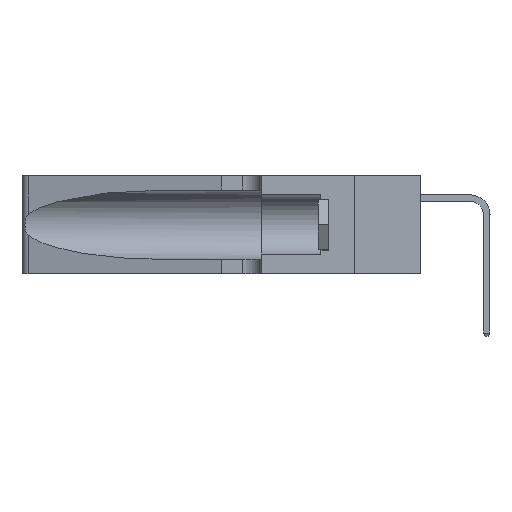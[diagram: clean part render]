
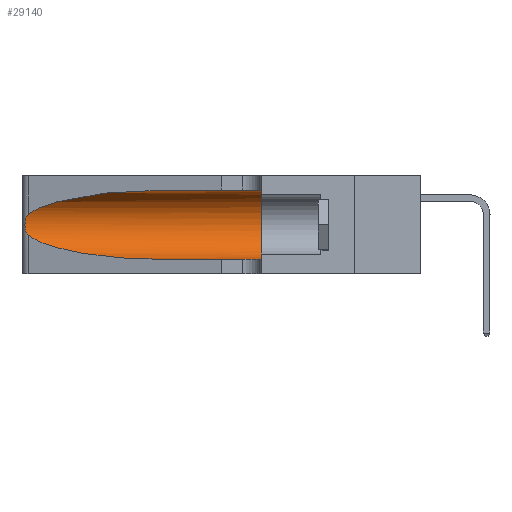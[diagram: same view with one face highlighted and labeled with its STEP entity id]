
A CAD part, left-side view. The second image highlights one B-rep face of the part: STEP entity #29140.
In plain terms, the highlighted cylindrical face has radius 3.308 mm (diameter 6.617 mm), a partial arc.
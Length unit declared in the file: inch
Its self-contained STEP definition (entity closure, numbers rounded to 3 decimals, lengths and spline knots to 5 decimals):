
#673 = CARTESIAN_POINT ( 'NONE',  ( 0.25487, 1.22718, 0.14631 ) ) ;
#947 = ORIENTED_EDGE ( 'NONE', *, *, #42946, .T. ) ;
#1863 = CARTESIAN_POINT ( 'NONE',  ( 0.1305, 0.35, 0.185 ) ) ;
#2248 = CARTESIAN_POINT ( 'NONE',  ( 0.25487, 1.22718, 0.22369 ) ) ;
#2252 = ORIENTED_EDGE ( 'NONE', *, *, #33688, .F. ) ;
#2518 = CARTESIAN_POINT ( 'NONE',  ( 0.1305, 1.61858, 0.05475 ) ) ;
#2894 = CARTESIAN_POINT ( 'NONE',  ( 0.18966, 0.96281, 0.31525 ) ) ;
#3070 = AXIS2_PLACEMENT_3D ( 'NONE', #3929, #15166, #40957 ) ;
#3604 = CARTESIAN_POINT ( 'NONE',  ( 0.26017, 1.23833, 0.17102 ) ) ;
#3897 = ORIENTED_EDGE ( 'NONE', *, *, #32656, .T. ) ;
#3929 = CARTESIAN_POINT ( 'NONE',  ( 0.1305, 1.61858, 0.185 ) ) ;
#5640 = DIRECTION ( 'NONE',  ( 0., 0., 1. ) ) ;
#5863 =( BOUNDED_CURVE ( )  B_SPLINE_CURVE ( 3, ( #28818, #2894, #32540, #10433 ),
 .UNSPECIFIED., .F., .T. ) 
 B_SPLINE_CURVE_WITH_KNOTS ( ( 4, 4 ),
 ( 1.5708, 2.84003 ),
 .UNSPECIFIED. ) 
 CURVE ( )  GEOMETRIC_REPRESENTATION_ITEM ( )  RATIONAL_B_SPLINE_CURVE ( ( 1., 0.87, 0.87, 1. ) ) 
 REPRESENTATION_ITEM ( '' )  );
#6295 = DIRECTION ( 'NONE',  ( 0., -1., 0. ) ) ;
#6692 = ORIENTED_EDGE ( 'NONE', *, *, #34399, .F. ) ;
#6877 = EDGE_CURVE ( 'NONE', #47892, #19113, #18857, .T. ) ;
#7237 = CARTESIAN_POINT ( 'NONE',  ( 0.25555, 1.22994, 0.2215 ) ) ;
#7405 = CARTESIAN_POINT ( 'NONE',  ( 0.25789, 1.23486, 0.15765 ) ) ;
#8239 = CARTESIAN_POINT ( 'NONE',  ( 0.1305, 0.72297, 0.05475 ) ) ;
#9835 = CARTESIAN_POINT ( 'NONE',  ( 0.1305, 1.61858, 0.31525 ) ) ;
#9887 = VECTOR ( 'NONE', #13546, 39.37008 ) ;
#10189 = EDGE_CURVE ( 'NONE', #40850, #20767, #39836, .T. ) ;
#10433 = CARTESIAN_POINT ( 'NONE',  ( 0.25487, 1.22718, 0.22369 ) ) ;
#11052 = LINE ( 'NONE', #9835, #9887 ) ;
#11140 = CARTESIAN_POINT ( 'NONE',  ( 0.25555, 1.22993, 0.14849 ) ) ;
#11400 = FACE_OUTER_BOUND ( 'NONE', #16375, .T. ) ;
#13546 = DIRECTION ( 'NONE',  ( 0., -1., 0. ) ) ;
#15166 = DIRECTION ( 'NONE',  ( 0., -1., 0. ) ) ;
#16375 = EDGE_LOOP ( 'NONE', ( #3897, #33234, #947, #39670, #2252, #6692 ) ) ;
#17641 = CARTESIAN_POINT ( 'NONE',  ( 0.1305, 0.35, 0.05475 ) ) ;
#17700 = VECTOR ( 'NONE', #6295, 39.37008 ) ;
#17708 = VERTEX_POINT ( 'NONE', #43520 ) ;
#18397 = CARTESIAN_POINT ( 'NONE',  ( 0.25787, 1.23484, 0.2124 ) ) ;
#18818 = CARTESIAN_POINT ( 'NONE',  ( 0.1305, 0.35, 0.31525 ) ) ;
#18857 = LINE ( 'NONE', #2518, #17700 ) ;
#19113 = VERTEX_POINT ( 'NONE', #17641 ) ;
#20767 = VERTEX_POINT ( 'NONE', #45323 ) ;
#22111 = CARTESIAN_POINT ( 'NONE',  ( 0.26018, 1.23835, 0.19895 ) ) ;
#25816 = CARTESIAN_POINT ( 'NONE',  ( 0.26075, 1.23896, 0.178 ) ) ;
#26641 = CARTESIAN_POINT ( 'NONE',  ( 0.2373, 1.15595, 0.08982 ) ) ;
#27815 = DIRECTION ( 'NONE',  ( 0., 1., 0. ) ) ;
#28818 = CARTESIAN_POINT ( 'NONE',  ( 0.1305, 0.72297, 0.31525 ) ) ;
#29140 = ADVANCED_FACE ( 'NONE', ( #11400 ), #38490, .F. ) ;
#29529 = CARTESIAN_POINT ( 'NONE',  ( 0.25856, 1.23593, 0.16098 ) ) ;
#30352 = CARTESIAN_POINT ( 'NONE',  ( 0.18966, 0.96281, 0.05475 ) ) ;
#32540 = CARTESIAN_POINT ( 'NONE',  ( 0.2373, 1.15595, 0.28018 ) ) ;
#32656 = EDGE_CURVE ( 'NONE', #17708, #40850, #5863, .T. ) ;
#33077 = CARTESIAN_POINT ( 'NONE',  ( 0.25639, 1.23184, 0.21858 ) ) ;
#33234 = ORIENTED_EDGE ( 'NONE', *, *, #10189, .T. ) ;
#33237 = CARTESIAN_POINT ( 'NONE',  ( 0.25639, 1.23186, 0.15144 ) ) ;
#33688 = EDGE_CURVE ( 'NONE', #38051, #19113, #41632, .T. ) ;
#34399 = EDGE_CURVE ( 'NONE', #17708, #38051, #11052, .T. ) ;
#35088 =( BOUNDED_CURVE ( )  B_SPLINE_CURVE ( 3, ( #673, #26641, #30352, #8239 ),
 .UNSPECIFIED., .F., .F. ) 
 B_SPLINE_CURVE_WITH_KNOTS ( ( 4, 4 ),
 ( 3.44316, 4.71239 ),
 .UNSPECIFIED. ) 
 CURVE ( )  GEOMETRIC_REPRESENTATION_ITEM ( )  RATIONAL_B_SPLINE_CURVE ( ( 1., 0.87, 0.87, 1. ) ) 
 REPRESENTATION_ITEM ( '' )  );
#36281 = CARTESIAN_POINT ( 'NONE',  ( 0.1305, 0.72297, 0.05475 ) ) ;
#36924 = CARTESIAN_POINT ( 'NONE',  ( 0.25487, 1.22718, 0.14631 ) ) ;
#38051 = VERTEX_POINT ( 'NONE', #18818 ) ;
#38490 = CYLINDRICAL_SURFACE ( 'NONE', #3070, 0.13025 ) ;
#39670 = ORIENTED_EDGE ( 'NONE', *, *, #6877, .T. ) ;
#39836 = B_SPLINE_CURVE_WITH_KNOTS ( 'NONE', 3,
 ( #40477, #7237, #33077, #18397, #44268, #22111, #48001, #25816, #3604, #29529, #7405, #33237, #11140, #36924 ),
 .UNSPECIFIED., .F., .F.,
 ( 4, 2, 2, 2, 2, 2, 4 ),
 ( 0., 0.00027, 0.00053, 0.00107, 0.0016, 0.00187, 0.00214 ),
 .UNSPECIFIED. ) ;
#40477 = CARTESIAN_POINT ( 'NONE',  ( 0.25487, 1.22718, 0.22369 ) ) ;
#40850 = VERTEX_POINT ( 'NONE', #2248 ) ;
#40957 = DIRECTION ( 'NONE',  ( 0., 0., -1. ) ) ;
#41632 = CIRCLE ( 'NONE', #45710, 0.13025 ) ;
#42946 = EDGE_CURVE ( 'NONE', #20767, #47892, #35088, .T. ) ;
#43520 = CARTESIAN_POINT ( 'NONE',  ( 0.1305, 0.72297, 0.31525 ) ) ;
#44268 = CARTESIAN_POINT ( 'NONE',  ( 0.25854, 1.2359, 0.20912 ) ) ;
#45323 = CARTESIAN_POINT ( 'NONE',  ( 0.25487, 1.22718, 0.14631 ) ) ;
#45710 = AXIS2_PLACEMENT_3D ( 'NONE', #1863, #27815, #5640 ) ;
#47892 = VERTEX_POINT ( 'NONE', #36281 ) ;
#48001 = CARTESIAN_POINT ( 'NONE',  ( 0.26075, 1.23896, 0.19203 ) ) ;
